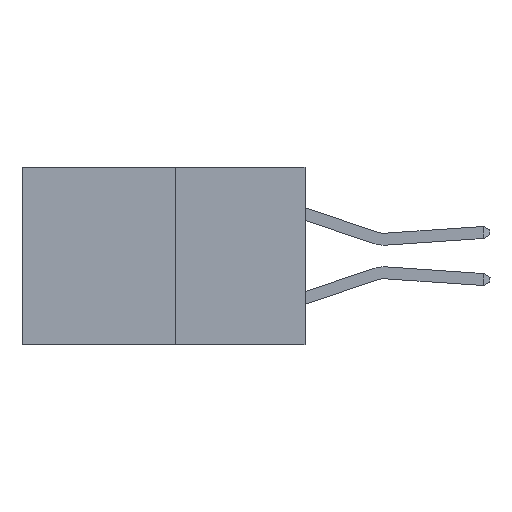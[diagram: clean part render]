
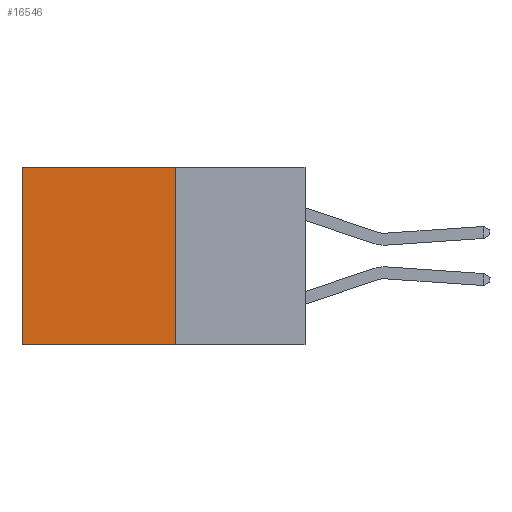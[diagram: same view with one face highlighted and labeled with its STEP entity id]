
A CAD part, left-side view. The second image highlights one B-rep face of the part: STEP entity #16546.
In plain terms, the highlighted planar face has unit normal (-1, 0, 0).
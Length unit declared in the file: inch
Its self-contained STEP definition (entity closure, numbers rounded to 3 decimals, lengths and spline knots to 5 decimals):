
#86 = DIRECTION ( 'NONE',  ( 0., 1., 0. ) ) ;
#268 = ORIENTED_EDGE ( 'NONE', *, *, #7309, .F. ) ;
#487 = ORIENTED_EDGE ( 'NONE', *, *, #7305, .F. ) ;
#2329 = VERTEX_POINT ( 'NONE', #15065 ) ;
#4102 = EDGE_LOOP ( 'NONE', ( #10616, #487, #268, #10978 ) ) ;
#5532 = DIRECTION ( 'NONE',  ( 0., 0., -1. ) ) ;
#5711 = AXIS2_PLACEMENT_3D ( 'NONE', #7017, #17393, #8494 ) ;
#5907 = CARTESIAN_POINT ( 'NONE',  ( 0.277, 0.27, -0.37 ) ) ;
#6397 = LINE ( 'NONE', #12536, #9396 ) ;
#6478 = VECTOR ( 'NONE', #5532, 39.37008 ) ;
#7017 = CARTESIAN_POINT ( 'NONE',  ( 0.277, 0.27, -0.37 ) ) ;
#7305 = EDGE_CURVE ( 'NONE', #11400, #15080, #13838, .T. ) ;
#7309 = EDGE_CURVE ( 'NONE', #15011, #11400, #6397, .T. ) ;
#8494 = DIRECTION ( 'NONE',  ( 0., 0., -1. ) ) ;
#9396 = VECTOR ( 'NONE', #12515, 39.37008 ) ;
#10488 = VECTOR ( 'NONE', #86, 39.37008 ) ;
#10616 = ORIENTED_EDGE ( 'NONE', *, *, #17335, .T. ) ;
#10792 = CARTESIAN_POINT ( 'NONE',  ( 0.277, 0.27, 0. ) ) ;
#10978 = ORIENTED_EDGE ( 'NONE', *, *, #16296, .T. ) ;
#11103 = CARTESIAN_POINT ( 'NONE',  ( 0.277, 0.27, 0. ) ) ;
#11400 = VERTEX_POINT ( 'NONE', #5907 ) ;
#11433 = CARTESIAN_POINT ( 'NONE',  ( 0.277, 0.59, -0.37 ) ) ;
#12515 = DIRECTION ( 'NONE',  ( 0., 0., -1. ) ) ;
#12536 = CARTESIAN_POINT ( 'NONE',  ( 0.277, 0.27, -0.37 ) ) ;
#12542 = CARTESIAN_POINT ( 'NONE',  ( 0.277, 0.27, -0.37 ) ) ;
#12809 = CARTESIAN_POINT ( 'NONE',  ( 0.277, 0.59, -0.37 ) ) ;
#12948 = PLANE ( 'NONE',  #5711 ) ;
#13000 = DIRECTION ( 'NONE',  ( 0., 1., 0. ) ) ;
#13369 = VECTOR ( 'NONE', #13000, 39.37008 ) ;
#13838 = LINE ( 'NONE', #12542, #13369 ) ;
#15011 = VERTEX_POINT ( 'NONE', #11103 ) ;
#15065 = CARTESIAN_POINT ( 'NONE',  ( 0.277, 0.59, 0. ) ) ;
#15080 = VERTEX_POINT ( 'NONE', #12809 ) ;
#16296 = EDGE_CURVE ( 'NONE', #15011, #2329, #17930, .T. ) ;
#16546 = ADVANCED_FACE ( 'NONE', ( #16841 ), #12948, .F. ) ;
#16841 = FACE_OUTER_BOUND ( 'NONE', #4102, .T. ) ;
#17335 = EDGE_CURVE ( 'NONE', #2329, #15080, #18733, .T. ) ;
#17393 = DIRECTION ( 'NONE',  ( 1., 0., 0. ) ) ;
#17930 = LINE ( 'NONE', #10792, #10488 ) ;
#18733 = LINE ( 'NONE', #11433, #6478 ) ;
